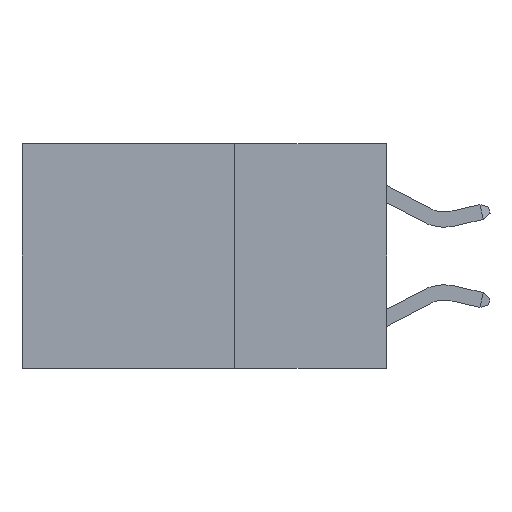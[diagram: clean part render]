
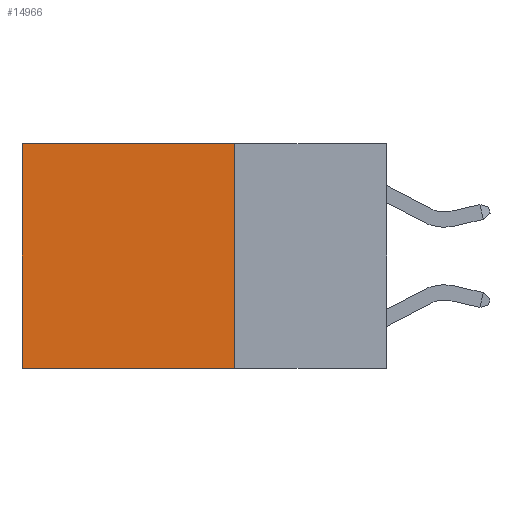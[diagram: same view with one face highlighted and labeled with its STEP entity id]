
A CAD part, left-side view. The second image highlights one B-rep face of the part: STEP entity #14966.
In plain terms, the highlighted planar face has unit normal (-1, 0, 0).
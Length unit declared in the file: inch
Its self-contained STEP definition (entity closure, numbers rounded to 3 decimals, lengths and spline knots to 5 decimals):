
#8 = DIRECTION ( 'NONE',  ( 0., 0., -1. ) ) ;
#85 = VERTEX_POINT ( 'NONE', #3828 ) ;
#870 = ORIENTED_EDGE ( 'NONE', *, *, #4595, .F. ) ;
#936 = FACE_OUTER_BOUND ( 'NONE', #15363, .T. ) ;
#2939 = VECTOR ( 'NONE', #15109, 39.37008 ) ;
#3828 = CARTESIAN_POINT ( 'NONE',  ( 0.2625, 0.25, 0. ) ) ;
#4595 = EDGE_CURVE ( 'NONE', #10644, #19069, #21097, .T. ) ;
#4890 = ORIENTED_EDGE ( 'NONE', *, *, #28987, .T. ) ;
#5154 = EDGE_CURVE ( 'NONE', #85, #15036, #17517, .T. ) ;
#5247 = DIRECTION ( 'NONE',  ( 1., 0., 0. ) ) ;
#5562 = LINE ( 'NONE', #11307, #6272 ) ;
#5584 = ORIENTED_EDGE ( 'NONE', *, *, #23172, .F. ) ;
#6272 = VECTOR ( 'NONE', #27225, 39.37008 ) ;
#6590 = AXIS2_PLACEMENT_3D ( 'NONE', #27904, #5247, #21169 ) ;
#9103 = CARTESIAN_POINT ( 'NONE',  ( 0.2625, 0.6, 0. ) ) ;
#9984 = CARTESIAN_POINT ( 'NONE',  ( 0.2625, 0.6, 0. ) ) ;
#10644 = VERTEX_POINT ( 'NONE', #18989 ) ;
#11307 = CARTESIAN_POINT ( 'NONE',  ( 0.2625, 0.25, 0. ) ) ;
#11999 = PLANE ( 'NONE',  #6590 ) ;
#14966 = ADVANCED_FACE ( 'NONE', ( #936 ), #11999, .F. ) ;
#15036 = VERTEX_POINT ( 'NONE', #9984 ) ;
#15109 = DIRECTION ( 'NONE',  ( 0., 1., 0. ) ) ;
#15363 = EDGE_LOOP ( 'NONE', ( #4890, #870, #5584, #28509 ) ) ;
#17517 = LINE ( 'NONE', #24234, #28848 ) ;
#18464 = LINE ( 'NONE', #9103, #23060 ) ;
#18989 = CARTESIAN_POINT ( 'NONE',  ( 0.2625, 0.25, -0.37 ) ) ;
#19069 = VERTEX_POINT ( 'NONE', #25511 ) ;
#21097 = LINE ( 'NONE', #26537, #2939 ) ;
#21169 = DIRECTION ( 'NONE',  ( 0., 0., -1. ) ) ;
#23060 = VECTOR ( 'NONE', #8, 39.37008 ) ;
#23172 = EDGE_CURVE ( 'NONE', #85, #10644, #5562, .T. ) ;
#24234 = CARTESIAN_POINT ( 'NONE',  ( 0.2625, 0.25, 0. ) ) ;
#25511 = CARTESIAN_POINT ( 'NONE',  ( 0.2625, 0.6, -0.37 ) ) ;
#26516 = DIRECTION ( 'NONE',  ( 0., 1., 0. ) ) ;
#26537 = CARTESIAN_POINT ( 'NONE',  ( 0.2625, 0.25, -0.37 ) ) ;
#27225 = DIRECTION ( 'NONE',  ( 0., 0., -1. ) ) ;
#27904 = CARTESIAN_POINT ( 'NONE',  ( 0.2625, 0.25, 0. ) ) ;
#28509 = ORIENTED_EDGE ( 'NONE', *, *, #5154, .T. ) ;
#28848 = VECTOR ( 'NONE', #26516, 39.37008 ) ;
#28987 = EDGE_CURVE ( 'NONE', #15036, #19069, #18464, .T. ) ;
